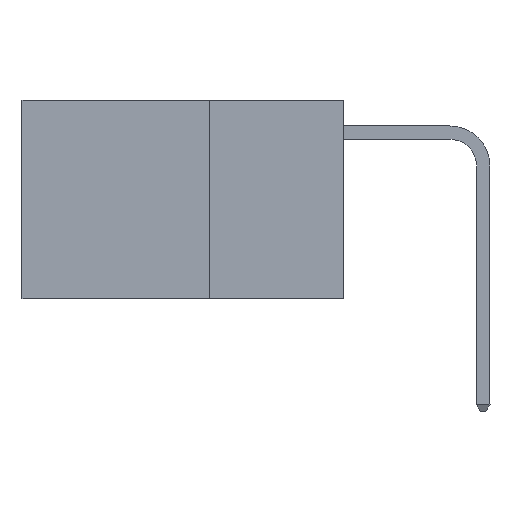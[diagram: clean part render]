
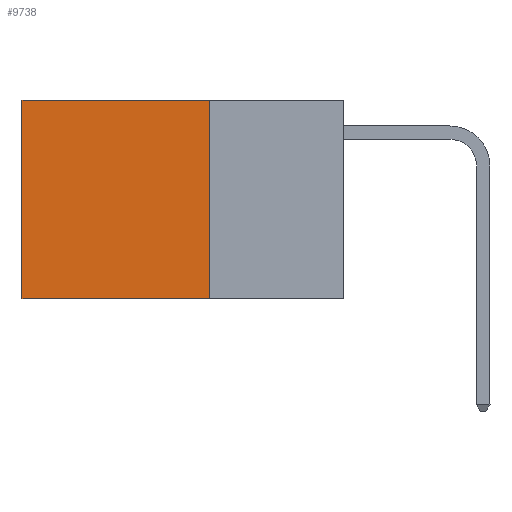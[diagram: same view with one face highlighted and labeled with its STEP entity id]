
A CAD part, left-side view. The second image highlights one B-rep face of the part: STEP entity #9738.
In plain terms, the highlighted planar face has unit normal (-1, 0, 0).
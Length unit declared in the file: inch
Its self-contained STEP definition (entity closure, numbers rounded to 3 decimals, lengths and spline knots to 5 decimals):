
#790 = ORIENTED_EDGE ( 'NONE', *, *, #10435, .T. ) ;
#1557 = CARTESIAN_POINT ( 'NONE',  ( 0.2625, 0.25, -0.37 ) ) ;
#1940 = CARTESIAN_POINT ( 'NONE',  ( 0.2625, 0.6, -0.37 ) ) ;
#2035 = ORIENTED_EDGE ( 'NONE', *, *, #2454, .F. ) ;
#2454 = EDGE_CURVE ( 'NONE', #12858, #3892, #15353, .T. ) ;
#2578 = VECTOR ( 'NONE', #15880, 39.37008 ) ;
#3892 = VERTEX_POINT ( 'NONE', #1940 ) ;
#4064 = ORIENTED_EDGE ( 'NONE', *, *, #14196, .F. ) ;
#5600 = VECTOR ( 'NONE', #15088, 39.37008 ) ;
#6504 = VECTOR ( 'NONE', #11849, 39.37008 ) ;
#7777 = LINE ( 'NONE', #13936, #19805 ) ;
#8380 = DIRECTION ( 'NONE',  ( 1., 0., 0. ) ) ;
#9138 = CARTESIAN_POINT ( 'NONE',  ( 0.2625, 0.25, -0.37 ) ) ;
#9738 = ADVANCED_FACE ( 'NONE', ( #13731 ), #19340, .F. ) ;
#9857 = EDGE_CURVE ( 'NONE', #18553, #3892, #15441, .T. ) ;
#9937 = CARTESIAN_POINT ( 'NONE',  ( 0.2625, 0.25, 0. ) ) ;
#10292 = CARTESIAN_POINT ( 'NONE',  ( 0.2625, 0.6, 0. ) ) ;
#10435 = EDGE_CURVE ( 'NONE', #16127, #18553, #7777, .T. ) ;
#10879 = DIRECTION ( 'NONE',  ( 0., 1., 0. ) ) ;
#11849 = DIRECTION ( 'NONE',  ( 0., 0., -1. ) ) ;
#11924 = CARTESIAN_POINT ( 'NONE',  ( 0.2625, 0.25, 0. ) ) ;
#12224 = CARTESIAN_POINT ( 'NONE',  ( 0.2625, 0.6, 0. ) ) ;
#12590 = ORIENTED_EDGE ( 'NONE', *, *, #9857, .T. ) ;
#12858 = VERTEX_POINT ( 'NONE', #9138 ) ;
#13086 = AXIS2_PLACEMENT_3D ( 'NONE', #9937, #8380, #19397 ) ;
#13731 = FACE_OUTER_BOUND ( 'NONE', #17402, .T. ) ;
#13936 = CARTESIAN_POINT ( 'NONE',  ( 0.2625, 0.25, 0. ) ) ;
#14196 = EDGE_CURVE ( 'NONE', #16127, #12858, #18279, .T. ) ;
#15088 = DIRECTION ( 'NONE',  ( 0., 0., -1. ) ) ;
#15353 = LINE ( 'NONE', #1557, #2578 ) ;
#15441 = LINE ( 'NONE', #10292, #6504 ) ;
#15880 = DIRECTION ( 'NONE',  ( 0., 1., 0. ) ) ;
#16127 = VERTEX_POINT ( 'NONE', #18544 ) ;
#17402 = EDGE_LOOP ( 'NONE', ( #12590, #2035, #4064, #790 ) ) ;
#18279 = LINE ( 'NONE', #11924, #5600 ) ;
#18544 = CARTESIAN_POINT ( 'NONE',  ( 0.2625, 0.25, 0. ) ) ;
#18553 = VERTEX_POINT ( 'NONE', #12224 ) ;
#19340 = PLANE ( 'NONE',  #13086 ) ;
#19397 = DIRECTION ( 'NONE',  ( 0., 0., -1. ) ) ;
#19805 = VECTOR ( 'NONE', #10879, 39.37008 ) ;
